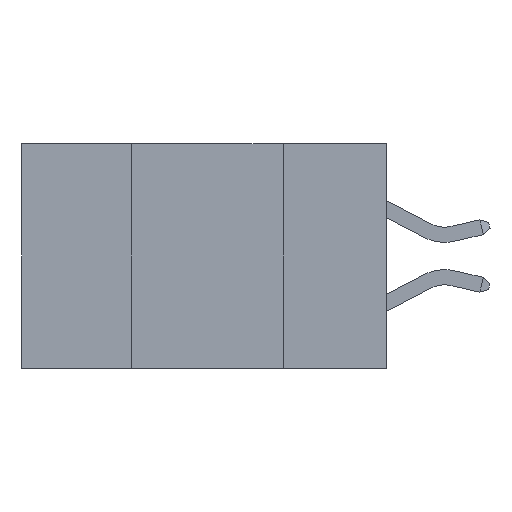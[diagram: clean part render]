
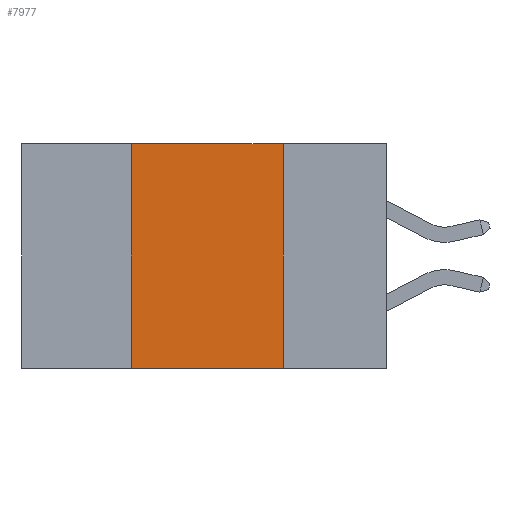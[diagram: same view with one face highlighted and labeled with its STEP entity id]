
A CAD part, left-side view. The second image highlights one B-rep face of the part: STEP entity #7977.
In plain terms, the highlighted planar face has unit normal (-1, 0, 0).
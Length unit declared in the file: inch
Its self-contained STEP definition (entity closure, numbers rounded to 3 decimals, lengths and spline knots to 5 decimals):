
#176 = ORIENTED_EDGE ( 'NONE', *, *, #19175, .T. ) ;
#824 = ORIENTED_EDGE ( 'NONE', *, *, #3678, .F. ) ;
#837 = VECTOR ( 'NONE', #1375, 39.37008 ) ;
#1290 = DIRECTION ( 'NONE',  ( 1., 0., 0. ) ) ;
#1303 = CARTESIAN_POINT ( 'NONE',  ( 0., 0.42, 0. ) ) ;
#1375 = DIRECTION ( 'NONE',  ( 0., 0., 1. ) ) ;
#1934 = LINE ( 'NONE', #5557, #10215 ) ;
#2095 = VERTEX_POINT ( 'NONE', #9094 ) ;
#3097 = LINE ( 'NONE', #12281, #15442 ) ;
#3678 = EDGE_CURVE ( 'NONE', #18257, #2095, #1934, .T. ) ;
#4790 = EDGE_CURVE ( 'NONE', #2095, #9222, #3097, .T. ) ;
#5473 = LINE ( 'NONE', #1303, #837 ) ;
#5557 = CARTESIAN_POINT ( 'NONE',  ( 0., 0.6, 0. ) ) ;
#5688 = DIRECTION ( 'NONE',  ( 0., 0., -1. ) ) ;
#6020 = LINE ( 'NONE', #6436, #17756 ) ;
#6254 = CARTESIAN_POINT ( 'NONE',  ( 0., 0.42, -0.37 ) ) ;
#6436 = CARTESIAN_POINT ( 'NONE',  ( 0., 0.6, -0.37 ) ) ;
#6863 = EDGE_CURVE ( 'NONE', #13264, #18257, #5473, .T. ) ;
#7512 = CARTESIAN_POINT ( 'NONE',  ( 0., 0.6, 0. ) ) ;
#7977 = ADVANCED_FACE ( 'NONE', ( #9309 ), #10548, .F. ) ;
#7985 = DIRECTION ( 'NONE',  ( 0., -1., 0. ) ) ;
#9094 = CARTESIAN_POINT ( 'NONE',  ( 0., 0.17, 0. ) ) ;
#9140 = EDGE_LOOP ( 'NONE', ( #15981, #824, #14980, #176 ) ) ;
#9222 = VERTEX_POINT ( 'NONE', #19420 ) ;
#9309 = FACE_OUTER_BOUND ( 'NONE', #9140, .T. ) ;
#10215 = VECTOR ( 'NONE', #18288, 39.37008 ) ;
#10548 = PLANE ( 'NONE',  #15856 ) ;
#12173 = DIRECTION ( 'NONE',  ( 0., 0., -1. ) ) ;
#12281 = CARTESIAN_POINT ( 'NONE',  ( 0., 0.17, 0. ) ) ;
#13264 = VERTEX_POINT ( 'NONE', #6254 ) ;
#13476 = CARTESIAN_POINT ( 'NONE',  ( 0., 0.42, 0. ) ) ;
#14980 = ORIENTED_EDGE ( 'NONE', *, *, #6863, .F. ) ;
#15442 = VECTOR ( 'NONE', #5688, 39.37008 ) ;
#15856 = AXIS2_PLACEMENT_3D ( 'NONE', #7512, #1290, #12173 ) ;
#15981 = ORIENTED_EDGE ( 'NONE', *, *, #4790, .F. ) ;
#17756 = VECTOR ( 'NONE', #7985, 39.37008 ) ;
#18257 = VERTEX_POINT ( 'NONE', #13476 ) ;
#18288 = DIRECTION ( 'NONE',  ( 0., -1., 0. ) ) ;
#19175 = EDGE_CURVE ( 'NONE', #13264, #9222, #6020, .T. ) ;
#19420 = CARTESIAN_POINT ( 'NONE',  ( 0., 0.17, -0.37 ) ) ;
